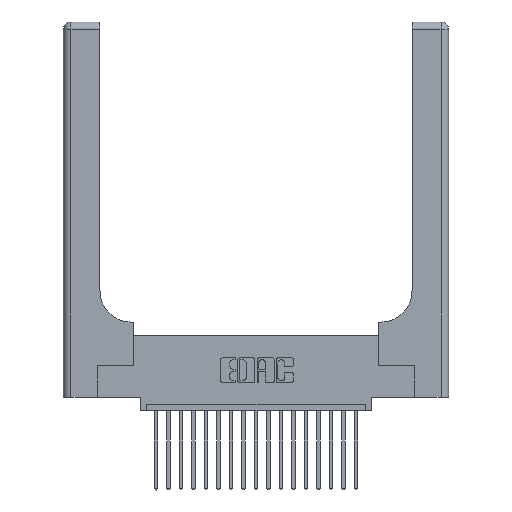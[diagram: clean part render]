
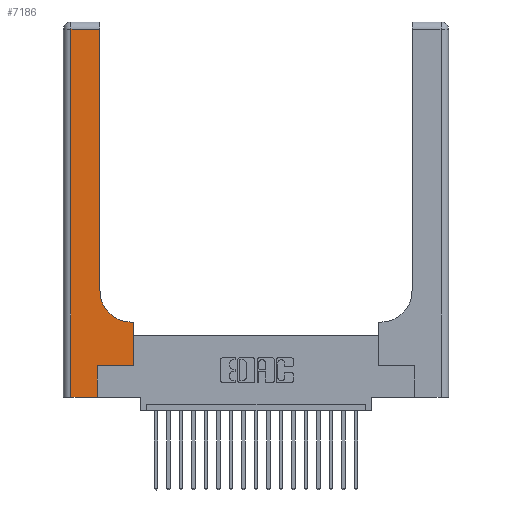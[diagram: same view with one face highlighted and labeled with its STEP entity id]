
A CAD part, top view. The second image highlights one B-rep face of the part: STEP entity #7186.
In plain terms, the highlighted planar face has unit normal (0, 0, 1).
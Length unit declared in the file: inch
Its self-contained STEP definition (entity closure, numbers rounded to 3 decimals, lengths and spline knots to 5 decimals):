
#2 = CARTESIAN_POINT ( 'NONE',  ( 0.269, 0.25, 0.37 ) ) ;
#210 = CARTESIAN_POINT ( 'NONE',  ( 0.5585, 0.25, 0.37 ) ) ;
#459 = VECTOR ( 'NONE', #20364, 39.37008 ) ;
#1632 = VERTEX_POINT ( 'NONE', #7414 ) ;
#1660 = CARTESIAN_POINT ( 'NONE',  ( 0., 0., 0.37 ) ) ;
#1716 = ORIENTED_EDGE ( 'NONE', *, *, #5705, .T. ) ;
#2127 = AXIS2_PLACEMENT_3D ( 'NONE', #2187, #4076, #7392 ) ;
#2187 = CARTESIAN_POINT ( 'NONE',  ( 0.5415, 0.85, 0.37 ) ) ;
#2234 = VERTEX_POINT ( 'NONE', #15530 ) ;
#2341 = VERTEX_POINT ( 'NONE', #17634 ) ;
#2549 = EDGE_CURVE ( 'NONE', #15230, #8192, #14480, .T. ) ;
#2693 = VERTEX_POINT ( 'NONE', #8695 ) ;
#2932 = ORIENTED_EDGE ( 'NONE', *, *, #7424, .T. ) ;
#2953 = PLANE ( 'NONE',  #16123 ) ;
#4076 = DIRECTION ( 'NONE',  ( 0., 0., -1. ) ) ;
#4261 = CARTESIAN_POINT ( 'NONE',  ( 0.06, 3., 0.37 ) ) ;
#4611 = DIRECTION ( 'NONE',  ( -1., 0., 0. ) ) ;
#4706 = EDGE_CURVE ( 'NONE', #18445, #2693, #16209, .T. ) ;
#5705 = EDGE_CURVE ( 'NONE', #2341, #1632, #15128, .T. ) ;
#5827 = CARTESIAN_POINT ( 'NONE',  ( 0.2915, 0.6, 0.37 ) ) ;
#6175 = ORIENTED_EDGE ( 'NONE', *, *, #8788, .T. ) ;
#7036 = CARTESIAN_POINT ( 'NONE',  ( 0.5585, 0.6, 0.37 ) ) ;
#7186 = ADVANCED_FACE ( 'NONE', ( #10794 ), #2953, .F. ) ;
#7392 = DIRECTION ( 'NONE',  ( 1., 0., 0. ) ) ;
#7414 = CARTESIAN_POINT ( 'NONE',  ( 0.06, 2.94, 0.37 ) ) ;
#7424 = EDGE_CURVE ( 'NONE', #2693, #2234, #18605, .T. ) ;
#7486 = ORIENTED_EDGE ( 'NONE', *, *, #2549, .T. ) ;
#7685 = EDGE_LOOP ( 'NONE', ( #20691, #1716, #20968, #19739, #2932, #13307, #7486, #6175, #11373 ) ) ;
#7741 = VECTOR ( 'NONE', #11637, 39.37008 ) ;
#7828 = CARTESIAN_POINT ( 'NONE',  ( 0.2915, 0.85, 0.37 ) ) ;
#8192 = VERTEX_POINT ( 'NONE', #7036 ) ;
#8695 = CARTESIAN_POINT ( 'NONE',  ( 0.269, 0., 0.37 ) ) ;
#8788 = EDGE_CURVE ( 'NONE', #8192, #15101, #18808, .T. ) ;
#8884 = VECTOR ( 'NONE', #10645, 39.37008 ) ;
#9880 = LINE ( 'NONE', #13891, #8884 ) ;
#10424 = VERTEX_POINT ( 'NONE', #7828 ) ;
#10547 = CARTESIAN_POINT ( 'NONE',  ( 0.5585, 0.25, 0.37 ) ) ;
#10645 = DIRECTION ( 'NONE',  ( 0., 1., 0. ) ) ;
#10794 = FACE_OUTER_BOUND ( 'NONE', #7685, .T. ) ;
#11052 = VECTOR ( 'NONE', #20928, 39.37008 ) ;
#11241 = CARTESIAN_POINT ( 'NONE',  ( 0., 3., 0.37 ) ) ;
#11373 = ORIENTED_EDGE ( 'NONE', *, *, #19662, .T. ) ;
#11402 = VECTOR ( 'NONE', #16780, 39.37008 ) ;
#11637 = DIRECTION ( 'NONE',  ( 1., 0., 0. ) ) ;
#11826 = VECTOR ( 'NONE', #15467, 39.37008 ) ;
#12133 = EDGE_CURVE ( 'NONE', #2234, #15230, #15995, .T. ) ;
#12679 = DIRECTION ( 'NONE',  ( 0., 0., -1. ) ) ;
#13217 = CARTESIAN_POINT ( 'NONE',  ( 0.269, 0., 0.37 ) ) ;
#13307 = ORIENTED_EDGE ( 'NONE', *, *, #12133, .T. ) ;
#13335 = VECTOR ( 'NONE', #19876, 39.37008 ) ;
#13891 = CARTESIAN_POINT ( 'NONE',  ( 0.2915, 3., 0.37 ) ) ;
#14426 = CARTESIAN_POINT ( 'NONE',  ( 0., 2.94, 0.37 ) ) ;
#14480 = LINE ( 'NONE', #210, #11402 ) ;
#14599 = CIRCLE ( 'NONE', #2127, 0.25 ) ;
#14856 = VECTOR ( 'NONE', #20636, 39.37008 ) ;
#14923 = EDGE_CURVE ( 'NONE', #10424, #2341, #9880, .T. ) ;
#15101 = VERTEX_POINT ( 'NONE', #19420 ) ;
#15128 = LINE ( 'NONE', #14426, #13335 ) ;
#15230 = VERTEX_POINT ( 'NONE', #10547 ) ;
#15467 = DIRECTION ( 'NONE',  ( 1., 0., 0. ) ) ;
#15530 = CARTESIAN_POINT ( 'NONE',  ( 0.269, 0.25, 0.37 ) ) ;
#15995 = LINE ( 'NONE', #2, #7741 ) ;
#16123 = AXIS2_PLACEMENT_3D ( 'NONE', #11241, #12679, #4611 ) ;
#16209 = LINE ( 'NONE', #1660, #11826 ) ;
#16780 = DIRECTION ( 'NONE',  ( 0., 1., 0. ) ) ;
#17622 = EDGE_CURVE ( 'NONE', #1632, #18445, #21482, .T. ) ;
#17634 = CARTESIAN_POINT ( 'NONE',  ( 0.2915, 2.94, 0.37 ) ) ;
#18445 = VERTEX_POINT ( 'NONE', #19940 ) ;
#18605 = LINE ( 'NONE', #13217, #459 ) ;
#18808 = LINE ( 'NONE', #5827, #14856 ) ;
#19420 = CARTESIAN_POINT ( 'NONE',  ( 0.5415, 0.6, 0.37 ) ) ;
#19662 = EDGE_CURVE ( 'NONE', #15101, #10424, #14599, .T. ) ;
#19739 = ORIENTED_EDGE ( 'NONE', *, *, #4706, .T. ) ;
#19876 = DIRECTION ( 'NONE',  ( -1., 0., 0. ) ) ;
#19940 = CARTESIAN_POINT ( 'NONE',  ( 0.06, 0., 0.37 ) ) ;
#20364 = DIRECTION ( 'NONE',  ( 0., 1., 0. ) ) ;
#20636 = DIRECTION ( 'NONE',  ( -1., 0., 0. ) ) ;
#20691 = ORIENTED_EDGE ( 'NONE', *, *, #14923, .T. ) ;
#20928 = DIRECTION ( 'NONE',  ( 0., -1., 0. ) ) ;
#20968 = ORIENTED_EDGE ( 'NONE', *, *, #17622, .T. ) ;
#21482 = LINE ( 'NONE', #4261, #11052 ) ;
